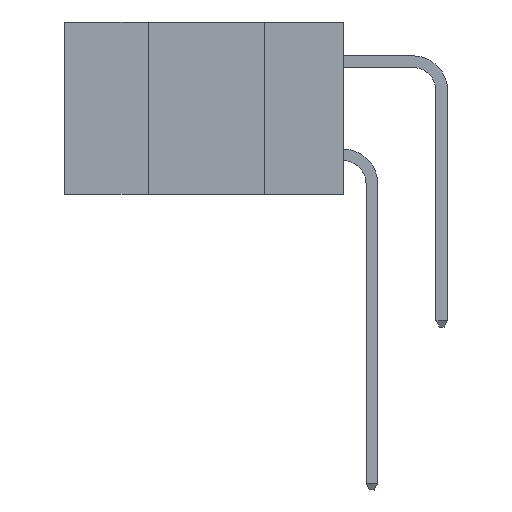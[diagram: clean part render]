
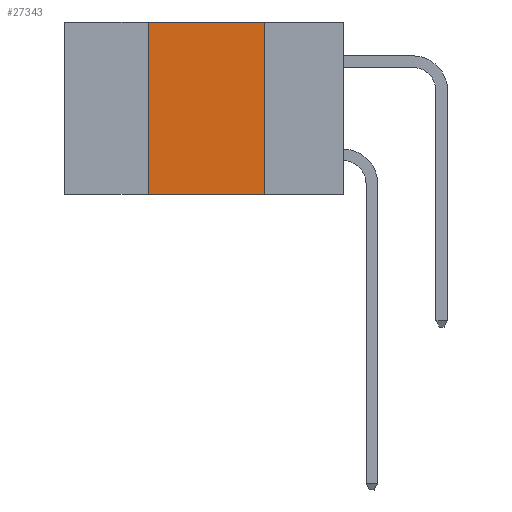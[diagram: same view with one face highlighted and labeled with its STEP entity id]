
A CAD part, left-side view. The second image highlights one B-rep face of the part: STEP entity #27343.
In plain terms, the highlighted planar face has unit normal (-1, 0, 0).
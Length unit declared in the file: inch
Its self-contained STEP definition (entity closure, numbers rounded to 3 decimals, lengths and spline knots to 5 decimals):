
#99 = DIRECTION ( 'NONE',  ( 0., 0., -1. ) ) ;
#1898 = LINE ( 'NONE', #27514, #23042 ) ;
#2378 = VERTEX_POINT ( 'NONE', #27492 ) ;
#3448 = EDGE_CURVE ( 'NONE', #18437, #8276, #5199, .T. ) ;
#3591 = DIRECTION ( 'NONE',  ( 0., -1., 0. ) ) ;
#3876 = FACE_OUTER_BOUND ( 'NONE', #16661, .T. ) ;
#4513 = VECTOR ( 'NONE', #22519, 39.37008 ) ;
#4535 = EDGE_CURVE ( 'NONE', #2378, #5980, #22247, .T. ) ;
#4963 = CARTESIAN_POINT ( 'NONE',  ( 0., 0.17, 0. ) ) ;
#5199 = LINE ( 'NONE', #4963, #4513 ) ;
#5566 = CARTESIAN_POINT ( 'NONE',  ( 0., 0.17, -0.37 ) ) ;
#5980 = VERTEX_POINT ( 'NONE', #13559 ) ;
#8276 = VERTEX_POINT ( 'NONE', #5566 ) ;
#8845 = PLANE ( 'NONE',  #25232 ) ;
#10688 = VECTOR ( 'NONE', #23135, 39.37008 ) ;
#12245 = EDGE_CURVE ( 'NONE', #5980, #18437, #1898, .T. ) ;
#13227 = DIRECTION ( 'NONE',  ( 1., 0., 0. ) ) ;
#13261 = CARTESIAN_POINT ( 'NONE',  ( 0., 0.42, 0. ) ) ;
#13559 = CARTESIAN_POINT ( 'NONE',  ( 0., 0.42, 0. ) ) ;
#14792 = VECTOR ( 'NONE', #3591, 39.37008 ) ;
#15885 = ORIENTED_EDGE ( 'NONE', *, *, #3448, .F. ) ;
#16661 = EDGE_LOOP ( 'NONE', ( #15885, #27736, #20736, #24546 ) ) ;
#18437 = VERTEX_POINT ( 'NONE', #23086 ) ;
#20570 = LINE ( 'NONE', #27378, #14792 ) ;
#20736 = ORIENTED_EDGE ( 'NONE', *, *, #4535, .F. ) ;
#21231 = EDGE_CURVE ( 'NONE', #2378, #8276, #20570, .T. ) ;
#22247 = LINE ( 'NONE', #13261, #10688 ) ;
#22519 = DIRECTION ( 'NONE',  ( 0., 0., -1. ) ) ;
#23042 = VECTOR ( 'NONE', #25412, 39.37008 ) ;
#23086 = CARTESIAN_POINT ( 'NONE',  ( 0., 0.17, 0. ) ) ;
#23135 = DIRECTION ( 'NONE',  ( 0., 0., 1. ) ) ;
#24546 = ORIENTED_EDGE ( 'NONE', *, *, #21231, .T. ) ;
#25232 = AXIS2_PLACEMENT_3D ( 'NONE', #26134, #13227, #99 ) ;
#25412 = DIRECTION ( 'NONE',  ( 0., -1., 0. ) ) ;
#26134 = CARTESIAN_POINT ( 'NONE',  ( 0., 0.6, 0. ) ) ;
#27343 = ADVANCED_FACE ( 'NONE', ( #3876 ), #8845, .F. ) ;
#27378 = CARTESIAN_POINT ( 'NONE',  ( 0., 0.6, -0.37 ) ) ;
#27492 = CARTESIAN_POINT ( 'NONE',  ( 0., 0.42, -0.37 ) ) ;
#27514 = CARTESIAN_POINT ( 'NONE',  ( 0., 0.6, 0. ) ) ;
#27736 = ORIENTED_EDGE ( 'NONE', *, *, #12245, .F. ) ;
